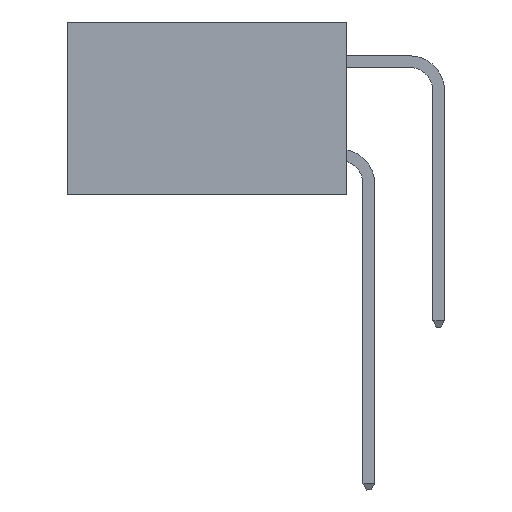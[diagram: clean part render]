
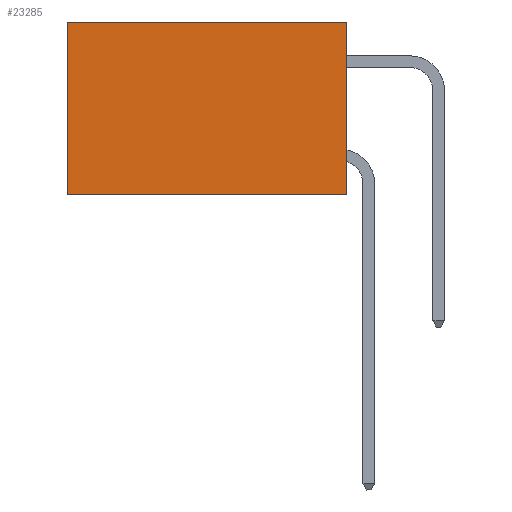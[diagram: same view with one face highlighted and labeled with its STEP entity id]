
A CAD part, left-side view. The second image highlights one B-rep face of the part: STEP entity #23285.
In plain terms, the highlighted planar face has unit normal (-1, 0, 0).
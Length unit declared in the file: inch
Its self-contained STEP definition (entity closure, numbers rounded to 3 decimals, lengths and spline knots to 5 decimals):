
#107 = EDGE_CURVE ( 'NONE', #2139, #18028, #2659, .T. ) ;
#148 = ORIENTED_EDGE ( 'NONE', *, *, #15143, .F. ) ;
#2139 = VERTEX_POINT ( 'NONE', #7460 ) ;
#2307 = VECTOR ( 'NONE', #9981, 39.37008 ) ;
#2407 = VERTEX_POINT ( 'NONE', #21152 ) ;
#2659 = LINE ( 'NONE', #7620, #11908 ) ;
#3906 = CARTESIAN_POINT ( 'NONE',  ( 0.2875, 0., 0. ) ) ;
#5276 = EDGE_CURVE ( 'NONE', #2407, #2139, #9216, .T. ) ;
#6125 = ORIENTED_EDGE ( 'NONE', *, *, #5276, .T. ) ;
#6938 = PLANE ( 'NONE',  #12202 ) ;
#7460 = CARTESIAN_POINT ( 'NONE',  ( 0.2875, 0.6, 0. ) ) ;
#7499 = DIRECTION ( 'NONE',  ( 0., 0., -1. ) ) ;
#7620 = CARTESIAN_POINT ( 'NONE',  ( 0.2875, 0.6, 0. ) ) ;
#8005 = VECTOR ( 'NONE', #8957, 39.37008 ) ;
#8957 = DIRECTION ( 'NONE',  ( 0., 1., 0. ) ) ;
#9216 = LINE ( 'NONE', #3906, #23306 ) ;
#9632 = VERTEX_POINT ( 'NONE', #17794 ) ;
#9981 = DIRECTION ( 'NONE',  ( 0., 0., -1. ) ) ;
#10637 = DIRECTION ( 'NONE',  ( 1., 0., 0. ) ) ;
#11675 = DIRECTION ( 'NONE',  ( 0., 1., 0. ) ) ;
#11908 = VECTOR ( 'NONE', #7499, 39.37008 ) ;
#12202 = AXIS2_PLACEMENT_3D ( 'NONE', #21697, #10637, #23497 ) ;
#12712 = LINE ( 'NONE', #13717, #2307 ) ;
#13717 = CARTESIAN_POINT ( 'NONE',  ( 0.2875, 0., 0. ) ) ;
#14450 = ORIENTED_EDGE ( 'NONE', *, *, #107, .T. ) ;
#14458 = FACE_OUTER_BOUND ( 'NONE', #19664, .T. ) ;
#14570 = CARTESIAN_POINT ( 'NONE',  ( 0.2875, 0., -0.37 ) ) ;
#15143 = EDGE_CURVE ( 'NONE', #2407, #9632, #12712, .T. ) ;
#17272 = CARTESIAN_POINT ( 'NONE',  ( 0.2875, 0.6, -0.37 ) ) ;
#17794 = CARTESIAN_POINT ( 'NONE',  ( 0.2875, 0., -0.37 ) ) ;
#17860 = LINE ( 'NONE', #14570, #8005 ) ;
#18028 = VERTEX_POINT ( 'NONE', #17272 ) ;
#18879 = EDGE_CURVE ( 'NONE', #9632, #18028, #17860, .T. ) ;
#19664 = EDGE_LOOP ( 'NONE', ( #14450, #22640, #148, #6125 ) ) ;
#21152 = CARTESIAN_POINT ( 'NONE',  ( 0.2875, 0., 0. ) ) ;
#21697 = CARTESIAN_POINT ( 'NONE',  ( 0.2875, 0., 0. ) ) ;
#22640 = ORIENTED_EDGE ( 'NONE', *, *, #18879, .F. ) ;
#23285 = ADVANCED_FACE ( 'NONE', ( #14458 ), #6938, .F. ) ;
#23306 = VECTOR ( 'NONE', #11675, 39.37008 ) ;
#23497 = DIRECTION ( 'NONE',  ( 0., 0., -1. ) ) ;
